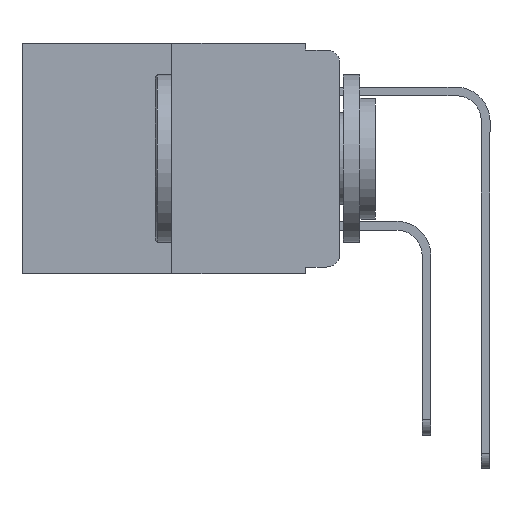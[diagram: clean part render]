
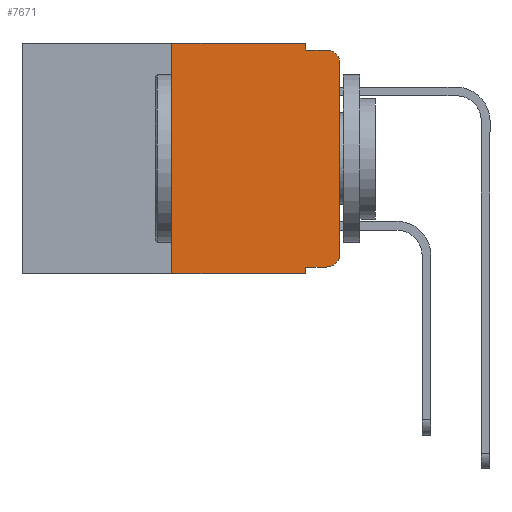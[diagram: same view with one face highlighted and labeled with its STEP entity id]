
A CAD part, left-side view. The second image highlights one B-rep face of the part: STEP entity #7671.
In plain terms, the highlighted planar face has unit normal (-1, 0, 0).
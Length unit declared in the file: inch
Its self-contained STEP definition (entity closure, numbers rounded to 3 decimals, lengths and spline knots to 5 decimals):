
#115 = DIRECTION ( 'NONE',  ( -1., 0., 0. ) ) ;
#444 = DIRECTION ( 'NONE',  ( 0., -1., 0. ) ) ;
#493 = ORIENTED_EDGE ( 'NONE', *, *, #7640, .T. ) ;
#616 = EDGE_CURVE ( 'NONE', #5903, #2193, #11845, .T. ) ;
#1108 = CARTESIAN_POINT ( 'NONE',  ( 0., 0.02, -0.01 ) ) ;
#1588 = CARTESIAN_POINT ( 'NONE',  ( 0., 0.473, -0.343 ) ) ;
#1868 = CARTESIAN_POINT ( 'NONE',  ( 0., 0.051, -0.01 ) ) ;
#1996 = VECTOR ( 'NONE', #5270, 39.37008 ) ;
#2193 = VERTEX_POINT ( 'NONE', #1108 ) ;
#2510 = LINE ( 'NONE', #3586, #13702 ) ;
#2538 = CARTESIAN_POINT ( 'NONE',  ( 0., 0.051, 0. ) ) ;
#2697 = LINE ( 'NONE', #8758, #3055 ) ;
#2782 = DIRECTION ( 'NONE',  ( -1., 0., 0. ) ) ;
#3055 = VECTOR ( 'NONE', #11944, 39.37008 ) ;
#3138 = LINE ( 'NONE', #5300, #12152 ) ;
#3233 = DIRECTION ( 'NONE',  ( 0., 0., -1. ) ) ;
#3294 = CARTESIAN_POINT ( 'NONE',  ( 0., 0.25, 0. ) ) ;
#3573 = CARTESIAN_POINT ( 'NONE',  ( 0., 0.473, 0. ) ) ;
#3586 = CARTESIAN_POINT ( 'NONE',  ( 0., 0.051, 0. ) ) ;
#4025 = FACE_OUTER_BOUND ( 'NONE', #4361, .T. ) ;
#4045 = ORIENTED_EDGE ( 'NONE', *, *, #13334, .F. ) ;
#4348 = CARTESIAN_POINT ( 'NONE',  ( 0., 0.02, -0.03 ) ) ;
#4361 = EDGE_LOOP ( 'NONE', ( #9201, #6668, #4045, #7015, #13005, #7677, #10857, #8693, #9030, #493 ) ) ;
#4397 = EDGE_CURVE ( 'NONE', #6559, #5903, #10782, .T. ) ;
#5000 = VECTOR ( 'NONE', #11185, 39.37008 ) ;
#5210 = CARTESIAN_POINT ( 'NONE',  ( 0., 0.02, -0.333 ) ) ;
#5270 = DIRECTION ( 'NONE',  ( 0., 0., 1. ) ) ;
#5300 = CARTESIAN_POINT ( 'NONE',  ( 0., 0.051, -0.01 ) ) ;
#5506 = VERTEX_POINT ( 'NONE', #7628 ) ;
#5826 = DIRECTION ( 'NONE',  ( 1., 0., 0. ) ) ;
#5903 = VERTEX_POINT ( 'NONE', #6291 ) ;
#6029 = VERTEX_POINT ( 'NONE', #5210 ) ;
#6291 = CARTESIAN_POINT ( 'NONE',  ( 0., 0., -0.03 ) ) ;
#6559 = VERTEX_POINT ( 'NONE', #11457 ) ;
#6668 = ORIENTED_EDGE ( 'NONE', *, *, #616, .T. ) ;
#6764 = AXIS2_PLACEMENT_3D ( 'NONE', #6908, #115, #7975 ) ;
#6908 = CARTESIAN_POINT ( 'NONE',  ( 0., 0.02, -0.313 ) ) ;
#6967 = DIRECTION ( 'NONE',  ( 0., 0., -1. ) ) ;
#7015 = ORIENTED_EDGE ( 'NONE', *, *, #12627, .F. ) ;
#7025 = LINE ( 'NONE', #9854, #10228 ) ;
#7628 = CARTESIAN_POINT ( 'NONE',  ( 0., 0.051, -0.333 ) ) ;
#7640 = EDGE_CURVE ( 'NONE', #6029, #6559, #10198, .T. ) ;
#7671 = ADVANCED_FACE ( 'NONE', ( #4025 ), #10162, .F. ) ;
#7677 = ORIENTED_EDGE ( 'NONE', *, *, #11920, .F. ) ;
#7975 = DIRECTION ( 'NONE',  ( 0., 0., -1. ) ) ;
#8235 = DIRECTION ( 'NONE',  ( 0., -1., 0. ) ) ;
#8608 = VERTEX_POINT ( 'NONE', #1868 ) ;
#8693 = ORIENTED_EDGE ( 'NONE', *, *, #11208, .F. ) ;
#8758 = CARTESIAN_POINT ( 'NONE',  ( 0., 0.473, 0. ) ) ;
#8822 = DIRECTION ( 'NONE',  ( 0., 0., -1. ) ) ;
#8939 = CARTESIAN_POINT ( 'NONE',  ( 0., 0.25, -0.343 ) ) ;
#9030 = ORIENTED_EDGE ( 'NONE', *, *, #9096, .T. ) ;
#9096 = EDGE_CURVE ( 'NONE', #5506, #6029, #14069, .T. ) ;
#9116 = VERTEX_POINT ( 'NONE', #13585 ) ;
#9201 = ORIENTED_EDGE ( 'NONE', *, *, #4397, .T. ) ;
#9854 = CARTESIAN_POINT ( 'NONE',  ( 0., 0.051, 0. ) ) ;
#9957 = CARTESIAN_POINT ( 'NONE',  ( 0., 0., 0. ) ) ;
#10162 = PLANE ( 'NONE',  #10384 ) ;
#10198 = CIRCLE ( 'NONE', #6764, 0.02 ) ;
#10228 = VECTOR ( 'NONE', #3233, 39.37008 ) ;
#10384 = AXIS2_PLACEMENT_3D ( 'NONE', #3573, #5826, #13309 ) ;
#10782 = LINE ( 'NONE', #9957, #5000 ) ;
#10857 = ORIENTED_EDGE ( 'NONE', *, *, #12310, .T. ) ;
#10988 = EDGE_CURVE ( 'NONE', #12063, #12897, #2697, .T. ) ;
#11185 = DIRECTION ( 'NONE',  ( 0., 0., 1. ) ) ;
#11208 = EDGE_CURVE ( 'NONE', #5506, #9116, #2510, .T. ) ;
#11354 = AXIS2_PLACEMENT_3D ( 'NONE', #4348, #2782, #8822 ) ;
#11356 = LINE ( 'NONE', #1588, #14149 ) ;
#11457 = CARTESIAN_POINT ( 'NONE',  ( 0., 0., -0.313 ) ) ;
#11758 = DIRECTION ( 'NONE',  ( 0., -1., 0. ) ) ;
#11845 = CIRCLE ( 'NONE', #11354, 0.02 ) ;
#11920 = EDGE_CURVE ( 'NONE', #13018, #12063, #13514, .T. ) ;
#11944 = DIRECTION ( 'NONE',  ( 0., -1., 0. ) ) ;
#12063 = VERTEX_POINT ( 'NONE', #3294 ) ;
#12152 = VECTOR ( 'NONE', #11758, 39.37008 ) ;
#12310 = EDGE_CURVE ( 'NONE', #13018, #9116, #11356, .T. ) ;
#12627 = EDGE_CURVE ( 'NONE', #12897, #8608, #7025, .T. ) ;
#12789 = CARTESIAN_POINT ( 'NONE',  ( 0., 0.25, 0. ) ) ;
#12897 = VERTEX_POINT ( 'NONE', #2538 ) ;
#13005 = ORIENTED_EDGE ( 'NONE', *, *, #10988, .F. ) ;
#13018 = VERTEX_POINT ( 'NONE', #8939 ) ;
#13309 = DIRECTION ( 'NONE',  ( 0., 0., -1. ) ) ;
#13334 = EDGE_CURVE ( 'NONE', #8608, #2193, #3138, .T. ) ;
#13514 = LINE ( 'NONE', #12789, #1996 ) ;
#13543 = CARTESIAN_POINT ( 'NONE',  ( 0., 0.051, -0.333 ) ) ;
#13585 = CARTESIAN_POINT ( 'NONE',  ( 0., 0.051, -0.343 ) ) ;
#13702 = VECTOR ( 'NONE', #6967, 39.37008 ) ;
#13744 = VECTOR ( 'NONE', #444, 39.37008 ) ;
#14069 = LINE ( 'NONE', #13543, #13744 ) ;
#14149 = VECTOR ( 'NONE', #8235, 39.37008 ) ;
